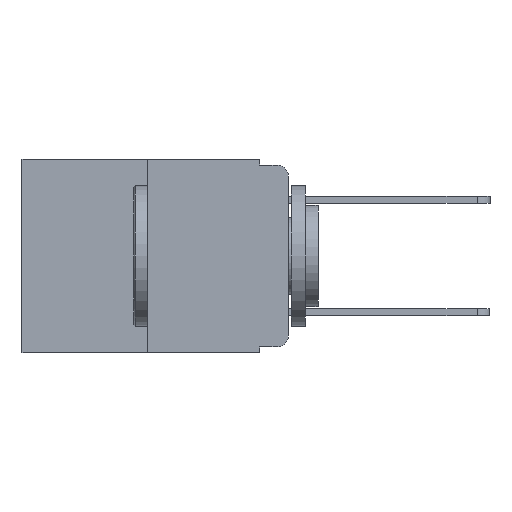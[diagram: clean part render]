
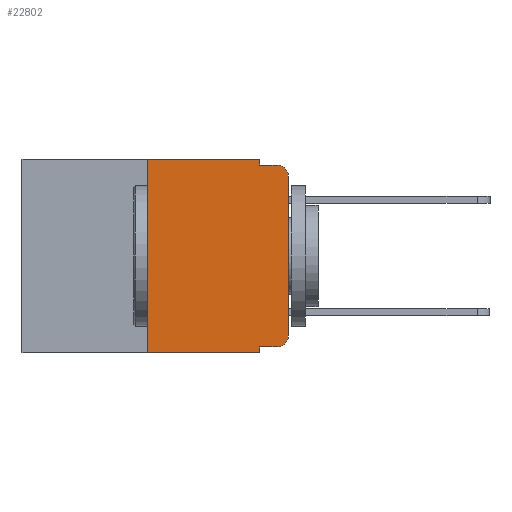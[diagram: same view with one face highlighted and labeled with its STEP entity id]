
A CAD part, left-side view. The second image highlights one B-rep face of the part: STEP entity #22802.
In plain terms, the highlighted planar face has unit normal (-1, 0, 0).
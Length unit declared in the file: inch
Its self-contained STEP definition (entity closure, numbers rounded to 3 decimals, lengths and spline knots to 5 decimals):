
#6 = CARTESIAN_POINT ( 'NONE',  ( 0., 0.02, -0.01 ) ) ;
#158 = VECTOR ( 'NONE', #11745, 39.37008 ) ;
#735 = VECTOR ( 'NONE', #23488, 39.37008 ) ;
#867 = CARTESIAN_POINT ( 'NONE',  ( 0., 0.051, -0.333 ) ) ;
#1106 = CARTESIAN_POINT ( 'NONE',  ( 0., 0.25, 0. ) ) ;
#1457 = CARTESIAN_POINT ( 'NONE',  ( 0., 0.051, 0. ) ) ;
#1952 = VERTEX_POINT ( 'NONE', #12683 ) ;
#2985 = VECTOR ( 'NONE', #21780, 39.37008 ) ;
#3046 = DIRECTION ( 'NONE',  ( 0., -1., 0. ) ) ;
#3376 = EDGE_CURVE ( 'NONE', #9457, #21797, #17608, .T. ) ;
#3520 = VECTOR ( 'NONE', #9378, 39.37008 ) ;
#3557 = DIRECTION ( 'NONE',  ( -1., 0., 0. ) ) ;
#3734 = CARTESIAN_POINT ( 'NONE',  ( 0., 0.051, -0.343 ) ) ;
#4660 = LINE ( 'NONE', #15324, #158 ) ;
#5096 = CARTESIAN_POINT ( 'NONE',  ( 0., 0.473, 0. ) ) ;
#5333 = ORIENTED_EDGE ( 'NONE', *, *, #13347, .T. ) ;
#5880 = EDGE_CURVE ( 'NONE', #13695, #13065, #17752, .T. ) ;
#6125 = LINE ( 'NONE', #867, #15374 ) ;
#6406 = LINE ( 'NONE', #10894, #735 ) ;
#6450 = VERTEX_POINT ( 'NONE', #1106 ) ;
#6750 = ORIENTED_EDGE ( 'NONE', *, *, #19773, .T. ) ;
#7036 = ORIENTED_EDGE ( 'NONE', *, *, #17012, .F. ) ;
#7161 = VECTOR ( 'NONE', #3046, 39.37008 ) ;
#7363 = CARTESIAN_POINT ( 'NONE',  ( 0., 0.02, -0.03 ) ) ;
#7509 = CARTESIAN_POINT ( 'NONE',  ( 0., 0.051, 0. ) ) ;
#8277 = VERTEX_POINT ( 'NONE', #6 ) ;
#8854 = ORIENTED_EDGE ( 'NONE', *, *, #5880, .F. ) ;
#9274 = DIRECTION ( 'NONE',  ( 0., 0., -1. ) ) ;
#9378 = DIRECTION ( 'NONE',  ( 0., 0., 1. ) ) ;
#9457 = VERTEX_POINT ( 'NONE', #20041 ) ;
#9930 = CARTESIAN_POINT ( 'NONE',  ( 0., 0.25, -0.343 ) ) ;
#10005 = ORIENTED_EDGE ( 'NONE', *, *, #11683, .F. ) ;
#10787 = PLANE ( 'NONE',  #18001 ) ;
#10891 = VERTEX_POINT ( 'NONE', #23191 ) ;
#10894 = CARTESIAN_POINT ( 'NONE',  ( 0., 0.051, 0. ) ) ;
#10988 = AXIS2_PLACEMENT_3D ( 'NONE', #14674, #3557, #16532 ) ;
#11629 = CARTESIAN_POINT ( 'NONE',  ( 0., 0.051, -0.333 ) ) ;
#11683 = EDGE_CURVE ( 'NONE', #15613, #6450, #17702, .T. ) ;
#11745 = DIRECTION ( 'NONE',  ( 0., 0., 1. ) ) ;
#12044 = VECTOR ( 'NONE', #17764, 39.37008 ) ;
#12405 = VERTEX_POINT ( 'NONE', #7509 ) ;
#12609 = DIRECTION ( 'NONE',  ( 0., 0., -1. ) ) ;
#12683 = CARTESIAN_POINT ( 'NONE',  ( 0., 0.051, -0.01 ) ) ;
#13065 = VERTEX_POINT ( 'NONE', #3734 ) ;
#13199 = EDGE_CURVE ( 'NONE', #21797, #10891, #4660, .T. ) ;
#13347 = EDGE_CURVE ( 'NONE', #13695, #9457, #6125, .T. ) ;
#13695 = VERTEX_POINT ( 'NONE', #11629 ) ;
#14180 = CARTESIAN_POINT ( 'NONE',  ( 0., 0.473, -0.343 ) ) ;
#14283 = LINE ( 'NONE', #23497, #18537 ) ;
#14554 = DIRECTION ( 'NONE',  ( 0., -1., 0. ) ) ;
#14674 = CARTESIAN_POINT ( 'NONE',  ( 0., 0.02, -0.313 ) ) ;
#15128 = ORIENTED_EDGE ( 'NONE', *, *, #22128, .F. ) ;
#15137 = ORIENTED_EDGE ( 'NONE', *, *, #19596, .F. ) ;
#15324 = CARTESIAN_POINT ( 'NONE',  ( 0., 0., 0. ) ) ;
#15374 = VECTOR ( 'NONE', #19382, 39.37008 ) ;
#15613 = VERTEX_POINT ( 'NONE', #9930 ) ;
#16340 = LINE ( 'NONE', #14180, #12044 ) ;
#16532 = DIRECTION ( 'NONE',  ( 0., 0., -1. ) ) ;
#16869 = CARTESIAN_POINT ( 'NONE',  ( 0., 0., -0.313 ) ) ;
#17012 = EDGE_CURVE ( 'NONE', #12405, #1952, #6406, .T. ) ;
#17608 = CIRCLE ( 'NONE', #10988, 0.02 ) ;
#17702 = LINE ( 'NONE', #20307, #3520 ) ;
#17752 = LINE ( 'NONE', #1457, #2985 ) ;
#17764 = DIRECTION ( 'NONE',  ( 0., -1., 0. ) ) ;
#17820 = CIRCLE ( 'NONE', #22557, 0.02 ) ;
#17821 = ORIENTED_EDGE ( 'NONE', *, *, #3376, .T. ) ;
#18001 = AXIS2_PLACEMENT_3D ( 'NONE', #5096, #23388, #12609 ) ;
#18214 = ORIENTED_EDGE ( 'NONE', *, *, #13199, .T. ) ;
#18537 = VECTOR ( 'NONE', #14554, 39.37008 ) ;
#18606 = FACE_OUTER_BOUND ( 'NONE', #18910, .T. ) ;
#18910 = EDGE_LOOP ( 'NONE', ( #18214, #6750, #15128, #7036, #15137, #10005, #23580, #8854, #5333, #17821 ) ) ;
#19382 = DIRECTION ( 'NONE',  ( 0., -1., 0. ) ) ;
#19596 = EDGE_CURVE ( 'NONE', #6450, #12405, #21742, .T. ) ;
#19608 = CARTESIAN_POINT ( 'NONE',  ( 0., 0.473, 0. ) ) ;
#19773 = EDGE_CURVE ( 'NONE', #10891, #8277, #17820, .T. ) ;
#20041 = CARTESIAN_POINT ( 'NONE',  ( 0., 0.02, -0.333 ) ) ;
#20213 = DIRECTION ( 'NONE',  ( -1., 0., 0. ) ) ;
#20307 = CARTESIAN_POINT ( 'NONE',  ( 0., 0.25, 0. ) ) ;
#21742 = LINE ( 'NONE', #19608, #7161 ) ;
#21780 = DIRECTION ( 'NONE',  ( 0., 0., -1. ) ) ;
#21797 = VERTEX_POINT ( 'NONE', #16869 ) ;
#22128 = EDGE_CURVE ( 'NONE', #1952, #8277, #14283, .T. ) ;
#22557 = AXIS2_PLACEMENT_3D ( 'NONE', #7363, #20213, #9274 ) ;
#22802 = ADVANCED_FACE ( 'NONE', ( #18606 ), #10787, .F. ) ;
#23191 = CARTESIAN_POINT ( 'NONE',  ( 0., 0., -0.03 ) ) ;
#23373 = EDGE_CURVE ( 'NONE', #15613, #13065, #16340, .T. ) ;
#23388 = DIRECTION ( 'NONE',  ( 1., 0., 0. ) ) ;
#23488 = DIRECTION ( 'NONE',  ( 0., 0., -1. ) ) ;
#23497 = CARTESIAN_POINT ( 'NONE',  ( 0., 0.051, -0.01 ) ) ;
#23580 = ORIENTED_EDGE ( 'NONE', *, *, #23373, .T. ) ;
